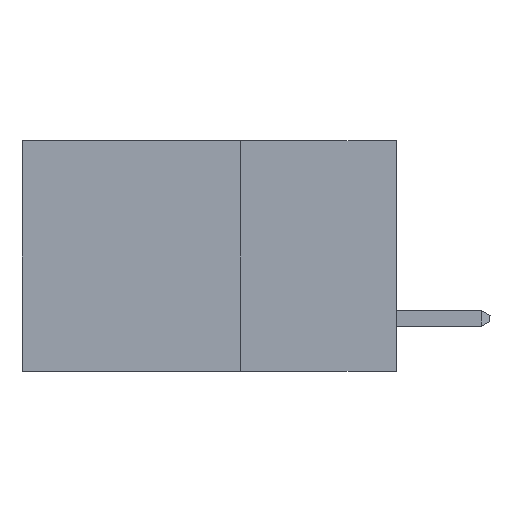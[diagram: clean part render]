
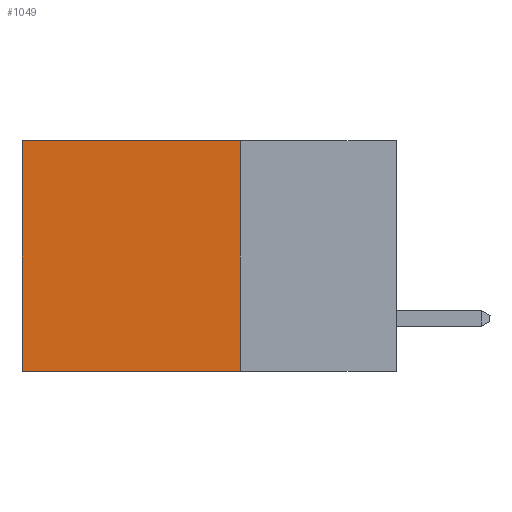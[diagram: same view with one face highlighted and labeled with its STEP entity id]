
A CAD part, left-side view. The second image highlights one B-rep face of the part: STEP entity #1049.
In plain terms, the highlighted planar face has unit normal (-1, 0, 0).
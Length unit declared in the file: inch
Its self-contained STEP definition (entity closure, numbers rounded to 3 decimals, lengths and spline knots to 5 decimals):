
#176 = DIRECTION ( 'NONE',  ( 0., 1., 0. ) ) ;
#1049 = ADVANCED_FACE ( 'NONE', ( #3006 ), #4262, .F. ) ;
#1187 = ORIENTED_EDGE ( 'NONE', *, *, #13444, .F. ) ;
#1708 = VERTEX_POINT ( 'NONE', #8252 ) ;
#1866 = CARTESIAN_POINT ( 'NONE',  ( 0.2615, 0.25, -0.37 ) ) ;
#2825 = CARTESIAN_POINT ( 'NONE',  ( 0.2615, 0.6, -0.37 ) ) ;
#2908 = DIRECTION ( 'NONE',  ( 0., 0., -1. ) ) ;
#2924 = DIRECTION ( 'NONE',  ( 0., 0., -1. ) ) ;
#3006 = FACE_OUTER_BOUND ( 'NONE', #4100, .T. ) ;
#3042 = DIRECTION ( 'NONE',  ( 0., 0., -1. ) ) ;
#4100 = EDGE_LOOP ( 'NONE', ( #12790, #1187, #10976, #12158 ) ) ;
#4262 = PLANE ( 'NONE',  #11627 ) ;
#5284 = DIRECTION ( 'NONE',  ( 1., 0., 0. ) ) ;
#6359 = LINE ( 'NONE', #1866, #13757 ) ;
#7691 = VERTEX_POINT ( 'NONE', #12865 ) ;
#8121 = VERTEX_POINT ( 'NONE', #13176 ) ;
#8252 = CARTESIAN_POINT ( 'NONE',  ( 0.2615, 0.6, -0.37 ) ) ;
#8488 = EDGE_CURVE ( 'NONE', #15482, #7691, #6359, .T. ) ;
#9451 = CARTESIAN_POINT ( 'NONE',  ( 0.2615, 0.25, 0. ) ) ;
#9821 = VECTOR ( 'NONE', #10630, 39.37008 ) ;
#9871 = CARTESIAN_POINT ( 'NONE',  ( 0.2615, 0.25, -0.37 ) ) ;
#10630 = DIRECTION ( 'NONE',  ( 0., 1., 0. ) ) ;
#10795 = VECTOR ( 'NONE', #176, 39.37008 ) ;
#10964 = LINE ( 'NONE', #9871, #10795 ) ;
#10976 = ORIENTED_EDGE ( 'NONE', *, *, #8488, .F. ) ;
#11627 = AXIS2_PLACEMENT_3D ( 'NONE', #12791, #5284, #2924 ) ;
#11808 = VECTOR ( 'NONE', #2908, 39.37008 ) ;
#12158 = ORIENTED_EDGE ( 'NONE', *, *, #12272, .T. ) ;
#12272 = EDGE_CURVE ( 'NONE', #15482, #8121, #15531, .T. ) ;
#12458 = LINE ( 'NONE', #2825, #11808 ) ;
#12790 = ORIENTED_EDGE ( 'NONE', *, *, #13425, .T. ) ;
#12791 = CARTESIAN_POINT ( 'NONE',  ( 0.2615, 0.25, -0.37 ) ) ;
#12865 = CARTESIAN_POINT ( 'NONE',  ( 0.2615, 0.25, -0.37 ) ) ;
#13008 = CARTESIAN_POINT ( 'NONE',  ( 0.2615, 0.25, 0. ) ) ;
#13176 = CARTESIAN_POINT ( 'NONE',  ( 0.2615, 0.6, 0. ) ) ;
#13425 = EDGE_CURVE ( 'NONE', #8121, #1708, #12458, .T. ) ;
#13444 = EDGE_CURVE ( 'NONE', #7691, #1708, #10964, .T. ) ;
#13757 = VECTOR ( 'NONE', #3042, 39.37008 ) ;
#15482 = VERTEX_POINT ( 'NONE', #9451 ) ;
#15531 = LINE ( 'NONE', #13008, #9821 ) ;
